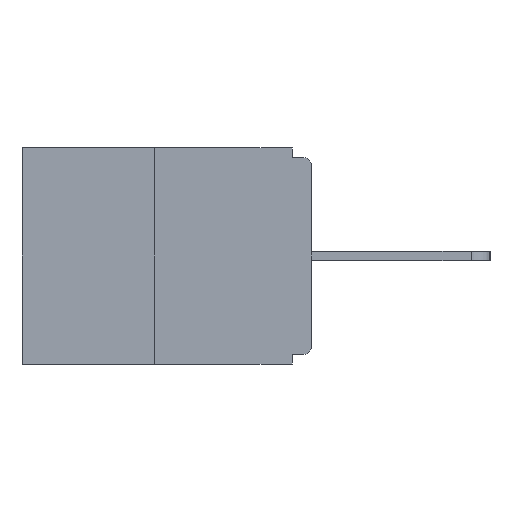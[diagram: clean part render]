
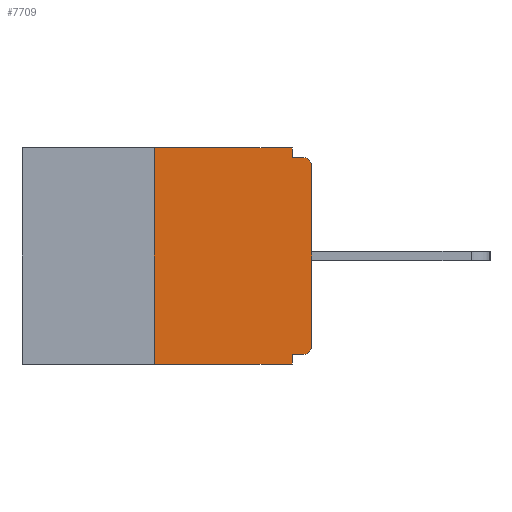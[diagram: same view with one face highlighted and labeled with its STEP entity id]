
A CAD part, left-side view. The second image highlights one B-rep face of the part: STEP entity #7709.
In plain terms, the highlighted planar face has unit normal (-1, 0, 0).
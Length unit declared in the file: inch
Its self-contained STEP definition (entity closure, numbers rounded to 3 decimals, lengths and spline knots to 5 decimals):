
#300 = CIRCLE ( 'NONE', #12892, 0.015 ) ;
#448 = CARTESIAN_POINT ( 'NONE',  ( 0., 0., -0.03 ) ) ;
#575 = DIRECTION ( 'NONE',  ( 0., -1., 0. ) ) ;
#599 = VECTOR ( 'NONE', #23946, 39.37008 ) ;
#615 = ORIENTED_EDGE ( 'NONE', *, *, #2443, .T. ) ;
#634 = CARTESIAN_POINT ( 'NONE',  ( 0., 0.031, -0.328 ) ) ;
#653 = DIRECTION ( 'NONE',  ( 0., -1., 0. ) ) ;
#1302 = EDGE_CURVE ( 'NONE', #12081, #23255, #19969, .T. ) ;
#1351 = CARTESIAN_POINT ( 'NONE',  ( 0., 0.015, -0.03 ) ) ;
#1550 = VERTEX_POINT ( 'NONE', #634 ) ;
#1998 = EDGE_CURVE ( 'NONE', #1550, #23255, #22781, .T. ) ;
#2097 = DIRECTION ( 'NONE',  ( 0., 0., -1. ) ) ;
#2181 = VERTEX_POINT ( 'NONE', #6646 ) ;
#2443 = EDGE_CURVE ( 'NONE', #4350, #14608, #21359, .T. ) ;
#3379 = CARTESIAN_POINT ( 'NONE',  ( 0., 0.015, -0.015 ) ) ;
#3721 = ORIENTED_EDGE ( 'NONE', *, *, #15168, .F. ) ;
#4188 = LINE ( 'NONE', #13505, #6670 ) ;
#4300 = ORIENTED_EDGE ( 'NONE', *, *, #1998, .F. ) ;
#4313 = ORIENTED_EDGE ( 'NONE', *, *, #9133, .F. ) ;
#4350 = VERTEX_POINT ( 'NONE', #7415 ) ;
#4380 = DIRECTION ( 'NONE',  ( 1., 0., 0. ) ) ;
#4485 = CARTESIAN_POINT ( 'NONE',  ( 0., 0., -0.328 ) ) ;
#4691 = EDGE_CURVE ( 'NONE', #12081, #13728, #8517, .T. ) ;
#4706 = DIRECTION ( 'NONE',  ( -1., 0., 0. ) ) ;
#4727 = DIRECTION ( 'NONE',  ( 0., 1., 0. ) ) ;
#5450 = CARTESIAN_POINT ( 'NONE',  ( 0., 0.25, 0. ) ) ;
#5797 = EDGE_CURVE ( 'NONE', #2181, #4350, #21052, .T. ) ;
#6646 = CARTESIAN_POINT ( 'NONE',  ( 0., 0.015, -0.328 ) ) ;
#6670 = VECTOR ( 'NONE', #7774, 39.37008 ) ;
#6718 = VERTEX_POINT ( 'NONE', #17019 ) ;
#6797 = DIRECTION ( 'NONE',  ( 0., 0., -1. ) ) ;
#6889 = CARTESIAN_POINT ( 'NONE',  ( 0., 0.25, 0. ) ) ;
#6964 = ORIENTED_EDGE ( 'NONE', *, *, #5797, .T. ) ;
#7415 = CARTESIAN_POINT ( 'NONE',  ( 0., 0., -0.313 ) ) ;
#7660 = CARTESIAN_POINT ( 'NONE',  ( 0., 0.031, -0.343 ) ) ;
#7709 = ADVANCED_FACE ( 'NONE', ( #19629 ), #13831, .F. ) ;
#7774 = DIRECTION ( 'NONE',  ( 0., 0., -1. ) ) ;
#8201 = LINE ( 'NONE', #4485, #21746 ) ;
#8517 = LINE ( 'NONE', #6889, #19454 ) ;
#9133 = EDGE_CURVE ( 'NONE', #13728, #12256, #16410, .T. ) ;
#9241 = AXIS2_PLACEMENT_3D ( 'NONE', #15438, #4380, #11952 ) ;
#10967 = LINE ( 'NONE', #17310, #13423 ) ;
#11429 = EDGE_CURVE ( 'NONE', #14608, #17480, #300, .T. ) ;
#11944 = AXIS2_PLACEMENT_3D ( 'NONE', #14850, #18547, #22522 ) ;
#11952 = DIRECTION ( 'NONE',  ( 0., 0., -1. ) ) ;
#12081 = VERTEX_POINT ( 'NONE', #24452 ) ;
#12256 = VERTEX_POINT ( 'NONE', #15799 ) ;
#12365 = VECTOR ( 'NONE', #20775, 39.37008 ) ;
#12565 = ORIENTED_EDGE ( 'NONE', *, *, #11429, .T. ) ;
#12892 = AXIS2_PLACEMENT_3D ( 'NONE', #1351, #4706, #6797 ) ;
#13248 = ORIENTED_EDGE ( 'NONE', *, *, #4691, .F. ) ;
#13423 = VECTOR ( 'NONE', #575, 39.37008 ) ;
#13505 = CARTESIAN_POINT ( 'NONE',  ( 0., 0.031, 0. ) ) ;
#13728 = VERTEX_POINT ( 'NONE', #5450 ) ;
#13831 = PLANE ( 'NONE',  #9241 ) ;
#14312 = CARTESIAN_POINT ( 'NONE',  ( 0., 0.46, 0. ) ) ;
#14473 = ORIENTED_EDGE ( 'NONE', *, *, #14578, .F. ) ;
#14478 = DIRECTION ( 'NONE',  ( 0., 0., 1. ) ) ;
#14578 = EDGE_CURVE ( 'NONE', #6718, #17480, #10967, .T. ) ;
#14608 = VERTEX_POINT ( 'NONE', #448 ) ;
#14850 = CARTESIAN_POINT ( 'NONE',  ( 0., 0.015, -0.313 ) ) ;
#15168 = EDGE_CURVE ( 'NONE', #2181, #1550, #8201, .T. ) ;
#15331 = VECTOR ( 'NONE', #653, 39.37008 ) ;
#15438 = CARTESIAN_POINT ( 'NONE',  ( 0., 0.46, 0. ) ) ;
#15799 = CARTESIAN_POINT ( 'NONE',  ( 0., 0.031, 0. ) ) ;
#16410 = LINE ( 'NONE', #14312, #599 ) ;
#17019 = CARTESIAN_POINT ( 'NONE',  ( 0., 0.031, -0.015 ) ) ;
#17310 = CARTESIAN_POINT ( 'NONE',  ( 0., 0., -0.015 ) ) ;
#17480 = VERTEX_POINT ( 'NONE', #3379 ) ;
#17633 = CARTESIAN_POINT ( 'NONE',  ( 0., 0.46, -0.343 ) ) ;
#18547 = DIRECTION ( 'NONE',  ( -1., 0., 0. ) ) ;
#19454 = VECTOR ( 'NONE', #14478, 39.37008 ) ;
#19491 = CARTESIAN_POINT ( 'NONE',  ( 0., 0., 0. ) ) ;
#19621 = EDGE_CURVE ( 'NONE', #12256, #6718, #4188, .T. ) ;
#19629 = FACE_OUTER_BOUND ( 'NONE', #20298, .T. ) ;
#19969 = LINE ( 'NONE', #17633, #15331 ) ;
#20039 = VECTOR ( 'NONE', #2097, 39.37008 ) ;
#20298 = EDGE_LOOP ( 'NONE', ( #4313, #13248, #22568, #4300, #3721, #6964, #615, #12565, #14473, #21472 ) ) ;
#20775 = DIRECTION ( 'NONE',  ( 0., 0., 1. ) ) ;
#21052 = CIRCLE ( 'NONE', #11944, 0.015 ) ;
#21359 = LINE ( 'NONE', #19491, #12365 ) ;
#21472 = ORIENTED_EDGE ( 'NONE', *, *, #19621, .F. ) ;
#21746 = VECTOR ( 'NONE', #4727, 39.37008 ) ;
#22522 = DIRECTION ( 'NONE',  ( 0., 0., -1. ) ) ;
#22568 = ORIENTED_EDGE ( 'NONE', *, *, #1302, .T. ) ;
#22781 = LINE ( 'NONE', #7660, #20039 ) ;
#23255 = VERTEX_POINT ( 'NONE', #23936 ) ;
#23936 = CARTESIAN_POINT ( 'NONE',  ( 0., 0.031, -0.343 ) ) ;
#23946 = DIRECTION ( 'NONE',  ( 0., -1., 0. ) ) ;
#24452 = CARTESIAN_POINT ( 'NONE',  ( 0., 0.25, -0.343 ) ) ;
